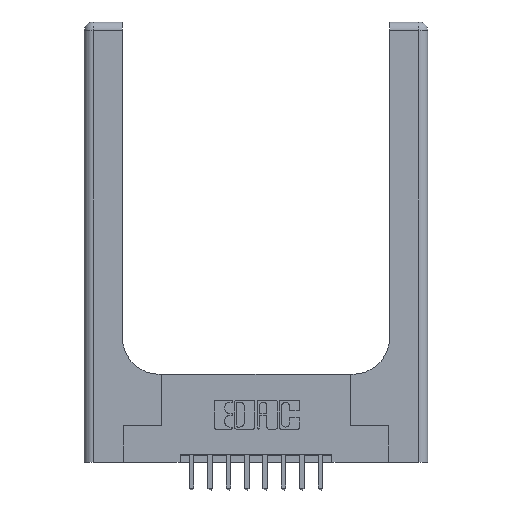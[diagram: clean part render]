
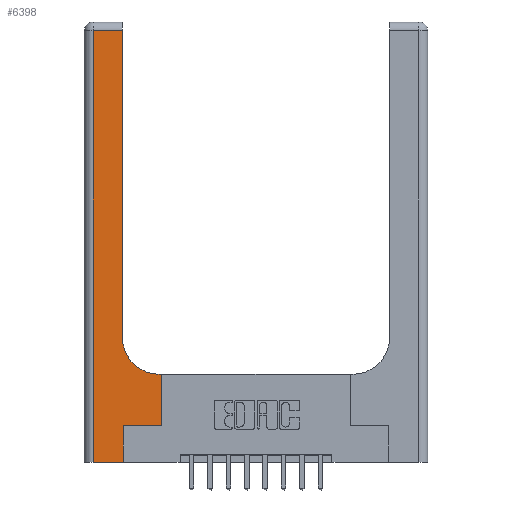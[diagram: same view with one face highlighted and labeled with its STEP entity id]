
A CAD part, top view. The second image highlights one B-rep face of the part: STEP entity #6398.
In plain terms, the highlighted planar face has unit normal (0, 0, 1).
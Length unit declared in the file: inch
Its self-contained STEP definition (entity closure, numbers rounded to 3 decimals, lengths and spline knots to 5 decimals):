
#751 = CARTESIAN_POINT ( 'NONE',  ( 0.265, 0.25, 0.37 ) ) ;
#1001 = DIRECTION ( 'NONE',  ( 1., 0., 0. ) ) ;
#1037 = CARTESIAN_POINT ( 'NONE',  ( 0.26, 0.6, 0.37 ) ) ;
#1074 = VECTOR ( 'NONE', #1001, 39.37008 ) ;
#1299 = VECTOR ( 'NONE', #14389, 39.37008 ) ;
#1505 = ORIENTED_EDGE ( 'NONE', *, *, #5324, .T. ) ;
#1749 = CARTESIAN_POINT ( 'NONE',  ( 0.06, 2.94, 0.37 ) ) ;
#1815 = FACE_OUTER_BOUND ( 'NONE', #14846, .T. ) ;
#1990 = VERTEX_POINT ( 'NONE', #3022 ) ;
#2047 = CARTESIAN_POINT ( 'NONE',  ( 0.06, 0., 0.37 ) ) ;
#2305 = VECTOR ( 'NONE', #12622, 39.37008 ) ;
#2557 = DIRECTION ( 'NONE',  ( 0., 0., -1. ) ) ;
#2728 = DIRECTION ( 'NONE',  ( 0., -1., 0. ) ) ;
#2815 = EDGE_CURVE ( 'NONE', #15219, #6558, #7251, .T. ) ;
#2914 = EDGE_CURVE ( 'NONE', #6558, #1990, #6659, .T. ) ;
#3011 = ORIENTED_EDGE ( 'NONE', *, *, #2914, .T. ) ;
#3022 = CARTESIAN_POINT ( 'NONE',  ( 0.26, 0.85, 0.37 ) ) ;
#3059 = ORIENTED_EDGE ( 'NONE', *, *, #15336, .T. ) ;
#3096 = VECTOR ( 'NONE', #7011, 39.37008 ) ;
#3140 = AXIS2_PLACEMENT_3D ( 'NONE', #15244, #6672, #4283 ) ;
#3557 = ORIENTED_EDGE ( 'NONE', *, *, #2815, .T. ) ;
#3711 = VERTEX_POINT ( 'NONE', #12719 ) ;
#3715 = DIRECTION ( 'NONE',  ( 0., 1., 0. ) ) ;
#3776 = CARTESIAN_POINT ( 'NONE',  ( 0.26, 3., 0.37 ) ) ;
#4283 = DIRECTION ( 'NONE',  ( -1., 0., 0. ) ) ;
#5025 = DIRECTION ( 'NONE',  ( 0., 1., 0. ) ) ;
#5135 = VERTEX_POINT ( 'NONE', #1749 ) ;
#5242 = VERTEX_POINT ( 'NONE', #2047 ) ;
#5324 = EDGE_CURVE ( 'NONE', #10954, #12253, #12522, .T. ) ;
#5591 = CARTESIAN_POINT ( 'NONE',  ( 0.265, 0.25, 0.37 ) ) ;
#5651 = CARTESIAN_POINT ( 'NONE',  ( 0.528, 0.6, 0.37 ) ) ;
#5988 = EDGE_CURVE ( 'NONE', #5242, #10954, #7215, .T. ) ;
#5997 = LINE ( 'NONE', #11824, #1299 ) ;
#6339 = LINE ( 'NONE', #11696, #2305 ) ;
#6398 = ADVANCED_FACE ( 'NONE', ( #1815 ), #14955, .F. ) ;
#6558 = VERTEX_POINT ( 'NONE', #10734 ) ;
#6632 = LINE ( 'NONE', #751, #10855 ) ;
#6659 = CIRCLE ( 'NONE', #12902, 0.25 ) ;
#6672 = DIRECTION ( 'NONE',  ( 0., 0., -1. ) ) ;
#7011 = DIRECTION ( 'NONE',  ( -1., 0., 0. ) ) ;
#7215 = LINE ( 'NONE', #9641, #1074 ) ;
#7251 = LINE ( 'NONE', #1037, #3096 ) ;
#7268 = ORIENTED_EDGE ( 'NONE', *, *, #13760, .T. ) ;
#7491 = DIRECTION ( 'NONE',  ( 1., 0., 0. ) ) ;
#7493 = VECTOR ( 'NONE', #2728, 39.37008 ) ;
#7511 = ORIENTED_EDGE ( 'NONE', *, *, #9315, .T. ) ;
#7680 = ORIENTED_EDGE ( 'NONE', *, *, #12108, .T. ) ;
#7926 = DIRECTION ( 'NONE',  ( 1., 0., 0. ) ) ;
#8363 = CARTESIAN_POINT ( 'NONE',  ( 0.265, 0., 0.37 ) ) ;
#8592 = EDGE_CURVE ( 'NONE', #13211, #5135, #5997, .T. ) ;
#8678 = LINE ( 'NONE', #12006, #7493 ) ;
#8847 = CARTESIAN_POINT ( 'NONE',  ( 0.51, 0.85, 0.37 ) ) ;
#9315 = EDGE_CURVE ( 'NONE', #12253, #3711, #6632, .T. ) ;
#9641 = CARTESIAN_POINT ( 'NONE',  ( 0., 0., 0.37 ) ) ;
#9709 = LINE ( 'NONE', #3776, #12205 ) ;
#10734 = CARTESIAN_POINT ( 'NONE',  ( 0.51, 0.6, 0.37 ) ) ;
#10855 = VECTOR ( 'NONE', #7926, 39.37008 ) ;
#10954 = VERTEX_POINT ( 'NONE', #8363 ) ;
#11161 = VECTOR ( 'NONE', #5025, 39.37008 ) ;
#11339 = CARTESIAN_POINT ( 'NONE',  ( 0.26, 2.94, 0.37 ) ) ;
#11696 = CARTESIAN_POINT ( 'NONE',  ( 0.528, 0.25, 0.37 ) ) ;
#11816 = ORIENTED_EDGE ( 'NONE', *, *, #8592, .T. ) ;
#11824 = CARTESIAN_POINT ( 'NONE',  ( 0., 2.94, 0.37 ) ) ;
#12006 = CARTESIAN_POINT ( 'NONE',  ( 0.06, 3., 0.37 ) ) ;
#12108 = EDGE_CURVE ( 'NONE', #1990, #13211, #9709, .T. ) ;
#12205 = VECTOR ( 'NONE', #3715, 39.37008 ) ;
#12253 = VERTEX_POINT ( 'NONE', #5591 ) ;
#12522 = LINE ( 'NONE', #15152, #11161 ) ;
#12622 = DIRECTION ( 'NONE',  ( 0., 1., 0. ) ) ;
#12719 = CARTESIAN_POINT ( 'NONE',  ( 0.528, 0.25, 0.37 ) ) ;
#12834 = ORIENTED_EDGE ( 'NONE', *, *, #5988, .T. ) ;
#12902 = AXIS2_PLACEMENT_3D ( 'NONE', #8847, #2557, #7491 ) ;
#13211 = VERTEX_POINT ( 'NONE', #11339 ) ;
#13760 = EDGE_CURVE ( 'NONE', #3711, #15219, #6339, .T. ) ;
#14389 = DIRECTION ( 'NONE',  ( -1., 0., 0. ) ) ;
#14846 = EDGE_LOOP ( 'NONE', ( #7680, #11816, #3059, #12834, #1505, #7511, #7268, #3557, #3011 ) ) ;
#14955 = PLANE ( 'NONE',  #3140 ) ;
#15152 = CARTESIAN_POINT ( 'NONE',  ( 0.265, 0., 0.37 ) ) ;
#15219 = VERTEX_POINT ( 'NONE', #5651 ) ;
#15244 = CARTESIAN_POINT ( 'NONE',  ( 0., 3., 0.37 ) ) ;
#15336 = EDGE_CURVE ( 'NONE', #5135, #5242, #8678, .T. ) ;
